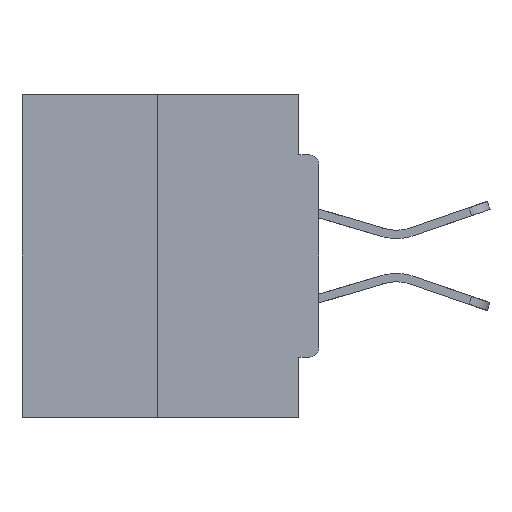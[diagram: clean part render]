
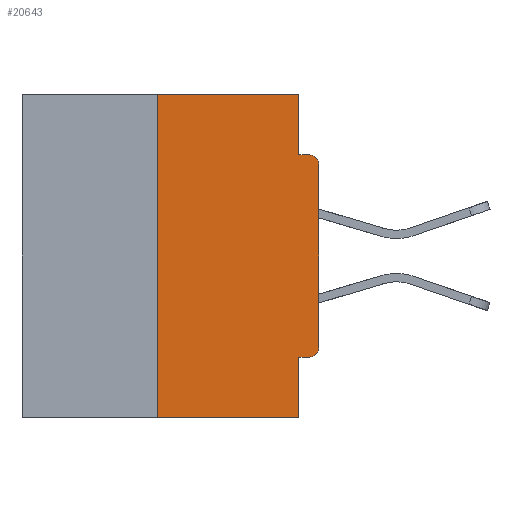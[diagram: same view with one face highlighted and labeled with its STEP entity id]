
A CAD part, left-side view. The second image highlights one B-rep face of the part: STEP entity #20643.
In plain terms, the highlighted planar face has unit normal (-1, 0, 0).
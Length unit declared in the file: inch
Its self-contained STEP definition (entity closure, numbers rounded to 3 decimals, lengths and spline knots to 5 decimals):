
#416 = EDGE_CURVE ( 'NONE', #6943, #24251, #26997, .T. ) ;
#1489 = EDGE_CURVE ( 'NONE', #30385, #20548, #8750, .T. ) ;
#1926 = EDGE_CURVE ( 'NONE', #3582, #22877, #4506, .T. ) ;
#1968 = CARTESIAN_POINT ( 'NONE',  ( 0., 0.031, 0. ) ) ;
#2259 = CARTESIAN_POINT ( 'NONE',  ( 0., 0.46, 0. ) ) ;
#3582 = VERTEX_POINT ( 'NONE', #13675 ) ;
#4506 = CIRCLE ( 'NONE', #12027, 0.015 ) ;
#4789 = CARTESIAN_POINT ( 'NONE',  ( 0., 0.46, -0.5 ) ) ;
#4884 = EDGE_CURVE ( 'NONE', #27397, #22814, #6975, .T. ) ;
#5155 = VECTOR ( 'NONE', #28524, 39.37008 ) ;
#5822 = DIRECTION ( 'NONE',  ( 0., -1., 0. ) ) ;
#6040 = VECTOR ( 'NONE', #32563, 39.37008 ) ;
#6363 = CARTESIAN_POINT ( 'NONE',  ( 0., 0.25, -0.5 ) ) ;
#6943 = VERTEX_POINT ( 'NONE', #1968 ) ;
#6975 = LINE ( 'NONE', #4789, #6040 ) ;
#7130 = VECTOR ( 'NONE', #18605, 39.37008 ) ;
#7461 = CARTESIAN_POINT ( 'NONE',  ( 0., 0.25, 0. ) ) ;
#7898 = AXIS2_PLACEMENT_3D ( 'NONE', #23644, #7912, #15436 ) ;
#7912 = DIRECTION ( 'NONE',  ( -1., 0., 0. ) ) ;
#8679 = DIRECTION ( 'NONE',  ( 0., 0., -1. ) ) ;
#8750 = LINE ( 'NONE', #28999, #5155 ) ;
#10829 = LINE ( 'NONE', #13676, #24026 ) ;
#10854 = VERTEX_POINT ( 'NONE', #29937 ) ;
#11651 = ORIENTED_EDGE ( 'NONE', *, *, #26369, .F. ) ;
#12027 = AXIS2_PLACEMENT_3D ( 'NONE', #31784, #13542, #8679 ) ;
#12106 = DIRECTION ( 'NONE',  ( 0., 0., -1. ) ) ;
#12993 = ORIENTED_EDGE ( 'NONE', *, *, #4884, .T. ) ;
#13542 = DIRECTION ( 'NONE',  ( -1., 0., 0. ) ) ;
#13675 = CARTESIAN_POINT ( 'NONE',  ( 0., 0., -0.1085 ) ) ;
#13676 = CARTESIAN_POINT ( 'NONE',  ( 0., 0., -0.0935 ) ) ;
#14404 = CARTESIAN_POINT ( 'NONE',  ( 0., 0., 0. ) ) ;
#15351 = ORIENTED_EDGE ( 'NONE', *, *, #1489, .F. ) ;
#15428 = ORIENTED_EDGE ( 'NONE', *, *, #21658, .F. ) ;
#15436 = DIRECTION ( 'NONE',  ( 0., 0., -1. ) ) ;
#16454 = DIRECTION ( 'NONE',  ( 0., 0., -1. ) ) ;
#16978 = CARTESIAN_POINT ( 'NONE',  ( 0., 0.015, -0.4065 ) ) ;
#17250 = EDGE_CURVE ( 'NONE', #24344, #6943, #26871, .T. ) ;
#17315 = DIRECTION ( 'NONE',  ( 1., 0., 0. ) ) ;
#17479 = ORIENTED_EDGE ( 'NONE', *, *, #21051, .F. ) ;
#17636 = VECTOR ( 'NONE', #24050, 39.37008 ) ;
#18093 = EDGE_CURVE ( 'NONE', #30385, #10854, #30869, .T. ) ;
#18605 = DIRECTION ( 'NONE',  ( 0., 0., 1. ) ) ;
#19632 = VECTOR ( 'NONE', #24623, 39.37008 ) ;
#19890 = CARTESIAN_POINT ( 'NONE',  ( 0., 0.031, -0.5 ) ) ;
#20410 = ORIENTED_EDGE ( 'NONE', *, *, #17250, .F. ) ;
#20548 = VERTEX_POINT ( 'NONE', #26853 ) ;
#20643 = ADVANCED_FACE ( 'NONE', ( #28016 ), #25008, .F. ) ;
#21015 = AXIS2_PLACEMENT_3D ( 'NONE', #2259, #17315, #12106 ) ;
#21051 = EDGE_CURVE ( 'NONE', #27397, #24344, #25988, .T. ) ;
#21367 = CARTESIAN_POINT ( 'NONE',  ( 0., 0.46, 0. ) ) ;
#21658 = EDGE_CURVE ( 'NONE', #20548, #22814, #23079, .T. ) ;
#21682 = ORIENTED_EDGE ( 'NONE', *, *, #18093, .T. ) ;
#22814 = VERTEX_POINT ( 'NONE', #19890 ) ;
#22877 = VERTEX_POINT ( 'NONE', #27590 ) ;
#23079 = LINE ( 'NONE', #25076, #23743 ) ;
#23644 = CARTESIAN_POINT ( 'NONE',  ( 0., 0.015, -0.3915 ) ) ;
#23743 = VECTOR ( 'NONE', #30602, 39.37008 ) ;
#24026 = VECTOR ( 'NONE', #5822, 39.37008 ) ;
#24050 = DIRECTION ( 'NONE',  ( 0., -1., 0. ) ) ;
#24251 = VERTEX_POINT ( 'NONE', #24381 ) ;
#24344 = VERTEX_POINT ( 'NONE', #7461 ) ;
#24381 = CARTESIAN_POINT ( 'NONE',  ( 0., 0.031, -0.0935 ) ) ;
#24518 = EDGE_CURVE ( 'NONE', #10854, #3582, #26620, .T. ) ;
#24623 = DIRECTION ( 'NONE',  ( 0., 0., 1. ) ) ;
#25008 = PLANE ( 'NONE',  #21015 ) ;
#25076 = CARTESIAN_POINT ( 'NONE',  ( 0., 0.031, -0.5 ) ) ;
#25988 = LINE ( 'NONE', #26310, #7130 ) ;
#26310 = CARTESIAN_POINT ( 'NONE',  ( 0., 0.25, 0. ) ) ;
#26369 = EDGE_CURVE ( 'NONE', #24251, #22877, #10829, .T. ) ;
#26620 = LINE ( 'NONE', #14404, #19632 ) ;
#26744 = ORIENTED_EDGE ( 'NONE', *, *, #24518, .T. ) ;
#26853 = CARTESIAN_POINT ( 'NONE',  ( 0., 0.031, -0.4065 ) ) ;
#26871 = LINE ( 'NONE', #21367, #17636 ) ;
#26997 = LINE ( 'NONE', #29328, #28621 ) ;
#27397 = VERTEX_POINT ( 'NONE', #6363 ) ;
#27590 = CARTESIAN_POINT ( 'NONE',  ( 0., 0.015, -0.0935 ) ) ;
#28016 = FACE_OUTER_BOUND ( 'NONE', #28409, .T. ) ;
#28409 = EDGE_LOOP ( 'NONE', ( #20410, #17479, #12993, #15428, #15351, #21682, #26744, #30494, #11651, #31551 ) ) ;
#28524 = DIRECTION ( 'NONE',  ( 0., 1., 0. ) ) ;
#28621 = VECTOR ( 'NONE', #16454, 39.37008 ) ;
#28999 = CARTESIAN_POINT ( 'NONE',  ( 0., 0., -0.4065 ) ) ;
#29328 = CARTESIAN_POINT ( 'NONE',  ( 0., 0.031, 0. ) ) ;
#29937 = CARTESIAN_POINT ( 'NONE',  ( 0., 0., -0.3915 ) ) ;
#30385 = VERTEX_POINT ( 'NONE', #16978 ) ;
#30494 = ORIENTED_EDGE ( 'NONE', *, *, #1926, .T. ) ;
#30602 = DIRECTION ( 'NONE',  ( 0., 0., -1. ) ) ;
#30869 = CIRCLE ( 'NONE', #7898, 0.015 ) ;
#31551 = ORIENTED_EDGE ( 'NONE', *, *, #416, .F. ) ;
#31784 = CARTESIAN_POINT ( 'NONE',  ( 0., 0.015, -0.1085 ) ) ;
#32563 = DIRECTION ( 'NONE',  ( 0., -1., 0. ) ) ;
